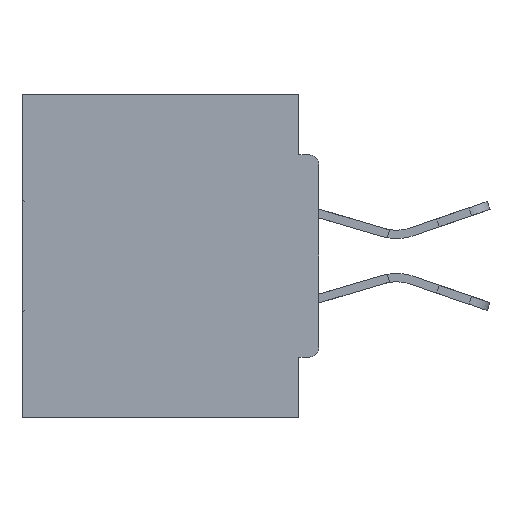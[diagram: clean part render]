
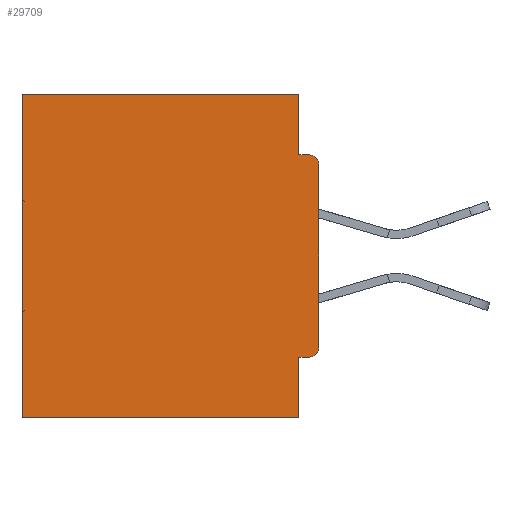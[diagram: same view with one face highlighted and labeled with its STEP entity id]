
A CAD part, left-side view. The second image highlights one B-rep face of the part: STEP entity #29709.
In plain terms, the highlighted planar face has unit normal (-1, 0, 0).
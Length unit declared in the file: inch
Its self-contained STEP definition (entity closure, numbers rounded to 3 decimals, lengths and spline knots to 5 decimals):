
#584 = VECTOR ( 'NONE', #24348, 39.37008 ) ;
#1404 = ORIENTED_EDGE ( 'NONE', *, *, #5550, .F. ) ;
#1439 = DIRECTION ( 'NONE',  ( 0., 0., -1. ) ) ;
#1453 = ORIENTED_EDGE ( 'NONE', *, *, #22192, .T. ) ;
#1466 = EDGE_CURVE ( 'NONE', #24995, #43304, #36661, .T. ) ;
#1516 = CARTESIAN_POINT ( 'NONE',  ( 0.298, 0.031, -0.5 ) ) ;
#1685 = EDGE_CURVE ( 'NONE', #7112, #22247, #9527, .T. ) ;
#1691 = AXIS2_PLACEMENT_3D ( 'NONE', #7460, #32253, #18050 ) ;
#1761 = LINE ( 'NONE', #33383, #32206 ) ;
#1878 = EDGE_LOOP ( 'NONE', ( #42397, #21047, #11543, #1453, #12992, #36863, #43445, #1404, #45479, #32798 ) ) ;
#3594 = CARTESIAN_POINT ( 'NONE',  ( 0.298, 0.015, -0.1085 ) ) ;
#3778 = EDGE_CURVE ( 'NONE', #7491, #7112, #44869, .T. ) ;
#4251 = CARTESIAN_POINT ( 'NONE',  ( 0.298, 0.031, -0.5 ) ) ;
#4735 = CARTESIAN_POINT ( 'NONE',  ( 0.298, 0.031, -0.5 ) ) ;
#4908 = LINE ( 'NONE', #10572, #36478 ) ;
#5229 = EDGE_CURVE ( 'NONE', #41833, #43304, #4908, .T. ) ;
#5322 = CARTESIAN_POINT ( 'NONE',  ( 0.298, 0.031, -0.4065 ) ) ;
#5550 = EDGE_CURVE ( 'NONE', #27932, #29103, #29809, .T. ) ;
#5596 = DIRECTION ( 'NONE',  ( 1., 0., 0. ) ) ;
#7112 = VERTEX_POINT ( 'NONE', #10878 ) ;
#7460 = CARTESIAN_POINT ( 'NONE',  ( 0.298, 0.015, -0.3915 ) ) ;
#7491 = VERTEX_POINT ( 'NONE', #45040 ) ;
#8602 = DIRECTION ( 'NONE',  ( 0., 0., -1. ) ) ;
#9527 = LINE ( 'NONE', #27359, #28848 ) ;
#10572 = CARTESIAN_POINT ( 'NONE',  ( 0.298, 0.46, 0. ) ) ;
#10713 = CARTESIAN_POINT ( 'NONE',  ( 0.298, 0., -0.4065 ) ) ;
#10878 = CARTESIAN_POINT ( 'NONE',  ( 0.298, 0.031, -0.0935 ) ) ;
#11543 = ORIENTED_EDGE ( 'NONE', *, *, #3778, .F. ) ;
#11664 = CARTESIAN_POINT ( 'NONE',  ( 0.298, 0., -0.5 ) ) ;
#12142 = DIRECTION ( 'NONE',  ( 0., 0., -1. ) ) ;
#12992 = ORIENTED_EDGE ( 'NONE', *, *, #5229, .T. ) ;
#13188 = VERTEX_POINT ( 'NONE', #43216 ) ;
#13215 = VECTOR ( 'NONE', #35830, 39.37008 ) ;
#13255 = CARTESIAN_POINT ( 'NONE',  ( 0.298, 0.46, -0.5 ) ) ;
#14255 = AXIS2_PLACEMENT_3D ( 'NONE', #3594, #31906, #38564 ) ;
#16056 = VECTOR ( 'NONE', #43749, 39.37008 ) ;
#16163 = CARTESIAN_POINT ( 'NONE',  ( 0.298, 0.015, -0.0935 ) ) ;
#17113 = EDGE_CURVE ( 'NONE', #13188, #22247, #29551, .T. ) ;
#18050 = DIRECTION ( 'NONE',  ( 0., 0., -1. ) ) ;
#19133 = EDGE_CURVE ( 'NONE', #27932, #26060, #45439, .T. ) ;
#19219 = VECTOR ( 'NONE', #28553, 39.37008 ) ;
#21047 = ORIENTED_EDGE ( 'NONE', *, *, #1685, .F. ) ;
#22192 = EDGE_CURVE ( 'NONE', #7491, #41833, #31627, .T. ) ;
#22247 = VERTEX_POINT ( 'NONE', #16163 ) ;
#23026 = PLANE ( 'NONE',  #45755 ) ;
#23399 = CARTESIAN_POINT ( 'NONE',  ( 0.298, 0.46, 0. ) ) ;
#24348 = DIRECTION ( 'NONE',  ( 0., 1., 0. ) ) ;
#24995 = VERTEX_POINT ( 'NONE', #4735 ) ;
#25506 = VECTOR ( 'NONE', #29506, 39.37008 ) ;
#26060 = VERTEX_POINT ( 'NONE', #44681 ) ;
#27359 = CARTESIAN_POINT ( 'NONE',  ( 0.298, 0., -0.0935 ) ) ;
#27932 = VERTEX_POINT ( 'NONE', #33829 ) ;
#28294 = EDGE_CURVE ( 'NONE', #29103, #24995, #45466, .T. ) ;
#28553 = DIRECTION ( 'NONE',  ( 0., 1., 0. ) ) ;
#28848 = VECTOR ( 'NONE', #34191, 39.37008 ) ;
#29103 = VERTEX_POINT ( 'NONE', #5322 ) ;
#29506 = DIRECTION ( 'NONE',  ( 0., 1., 0. ) ) ;
#29551 = CIRCLE ( 'NONE', #14255, 0.015 ) ;
#29709 = ADVANCED_FACE ( 'NONE', ( #41559 ), #23026, .F. ) ;
#29809 = LINE ( 'NONE', #10713, #19219 ) ;
#31353 = CARTESIAN_POINT ( 'NONE',  ( 0.298, 0., 0. ) ) ;
#31627 = LINE ( 'NONE', #31353, #584 ) ;
#31906 = DIRECTION ( 'NONE',  ( -1., 0., 0. ) ) ;
#32206 = VECTOR ( 'NONE', #8602, 39.37008 ) ;
#32253 = DIRECTION ( 'NONE',  ( -1., 0., 0. ) ) ;
#32798 = ORIENTED_EDGE ( 'NONE', *, *, #35047, .F. ) ;
#33383 = CARTESIAN_POINT ( 'NONE',  ( 0.298, 0., 0. ) ) ;
#33829 = CARTESIAN_POINT ( 'NONE',  ( 0.298, 0.015, -0.4065 ) ) ;
#34191 = DIRECTION ( 'NONE',  ( 0., -1., 0. ) ) ;
#35047 = EDGE_CURVE ( 'NONE', #13188, #26060, #1761, .T. ) ;
#35830 = DIRECTION ( 'NONE',  ( 0., 0., -1. ) ) ;
#36478 = VECTOR ( 'NONE', #1439, 39.37008 ) ;
#36661 = LINE ( 'NONE', #11664, #25506 ) ;
#36863 = ORIENTED_EDGE ( 'NONE', *, *, #1466, .F. ) ;
#38564 = DIRECTION ( 'NONE',  ( 0., 0., -1. ) ) ;
#40876 = CARTESIAN_POINT ( 'NONE',  ( 0.298, 0., 0. ) ) ;
#41559 = FACE_OUTER_BOUND ( 'NONE', #1878, .T. ) ;
#41833 = VERTEX_POINT ( 'NONE', #23399 ) ;
#42397 = ORIENTED_EDGE ( 'NONE', *, *, #17113, .T. ) ;
#43216 = CARTESIAN_POINT ( 'NONE',  ( 0.298, 0., -0.1085 ) ) ;
#43304 = VERTEX_POINT ( 'NONE', #13255 ) ;
#43445 = ORIENTED_EDGE ( 'NONE', *, *, #28294, .F. ) ;
#43749 = DIRECTION ( 'NONE',  ( 0., 0., -1. ) ) ;
#44681 = CARTESIAN_POINT ( 'NONE',  ( 0.298, 0., -0.3915 ) ) ;
#44869 = LINE ( 'NONE', #4251, #13215 ) ;
#45040 = CARTESIAN_POINT ( 'NONE',  ( 0.298, 0.031, 0. ) ) ;
#45439 = CIRCLE ( 'NONE', #1691, 0.015 ) ;
#45466 = LINE ( 'NONE', #1516, #16056 ) ;
#45479 = ORIENTED_EDGE ( 'NONE', *, *, #19133, .T. ) ;
#45755 = AXIS2_PLACEMENT_3D ( 'NONE', #40876, #5596, #12142 ) ;
